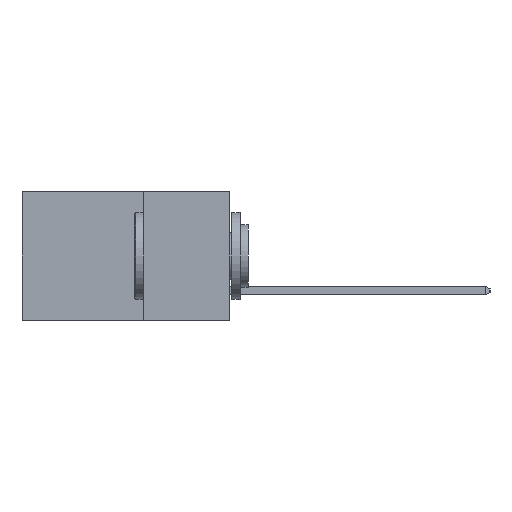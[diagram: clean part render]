
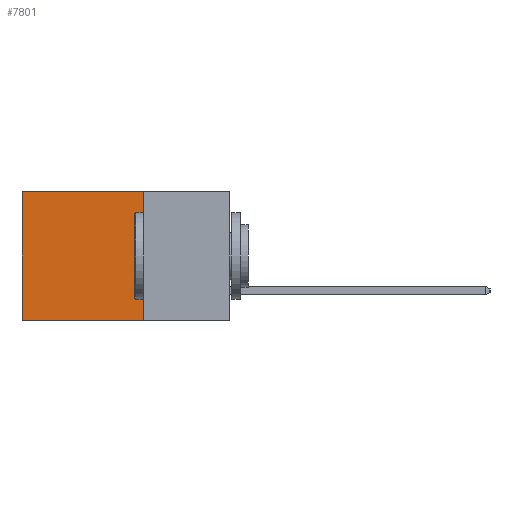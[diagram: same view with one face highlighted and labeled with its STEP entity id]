
A CAD part, left-side view. The second image highlights one B-rep face of the part: STEP entity #7801.
In plain terms, the highlighted planar face has unit normal (-1, 0, 0).
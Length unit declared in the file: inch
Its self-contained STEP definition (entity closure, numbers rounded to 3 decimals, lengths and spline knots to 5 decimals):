
#1 = LINE ( 'NONE', #16261, #3781 ) ;
#700 = ORIENTED_EDGE ( 'NONE', *, *, #13414, .F. ) ;
#1871 = ORIENTED_EDGE ( 'NONE', *, *, #15941, .T. ) ;
#2178 = CARTESIAN_POINT ( 'NONE',  ( 0.298, 0.25, 0. ) ) ;
#2342 = DIRECTION ( 'NONE',  ( 0., 0., -1. ) ) ;
#2393 = DIRECTION ( 'NONE',  ( 1., 0., 0. ) ) ;
#2459 = VECTOR ( 'NONE', #3857, 39.37008 ) ;
#2562 = CARTESIAN_POINT ( 'NONE',  ( 0.298, 0.25, 0. ) ) ;
#2691 = LINE ( 'NONE', #8338, #18317 ) ;
#3017 = PLANE ( 'NONE',  #8776 ) ;
#3781 = VECTOR ( 'NONE', #5329, 39.37008 ) ;
#3857 = DIRECTION ( 'NONE',  ( 0., 0., -1. ) ) ;
#3947 = CARTESIAN_POINT ( 'NONE',  ( 0.298, 0.6, 0. ) ) ;
#4878 = EDGE_LOOP ( 'NONE', ( #19168, #700, #9934, #1871 ) ) ;
#5329 = DIRECTION ( 'NONE',  ( 0., 1., 0. ) ) ;
#6420 = EDGE_CURVE ( 'NONE', #7809, #18587, #6676, .T. ) ;
#6676 = LINE ( 'NONE', #10028, #14474 ) ;
#7688 = EDGE_CURVE ( 'NONE', #8236, #14169, #10789, .T. ) ;
#7801 = ADVANCED_FACE ( 'NONE', ( #12972 ), #3017, .F. ) ;
#7809 = VERTEX_POINT ( 'NONE', #2178 ) ;
#8236 = VERTEX_POINT ( 'NONE', #13183 ) ;
#8338 = CARTESIAN_POINT ( 'NONE',  ( 0.298, 0.25, 0. ) ) ;
#8776 = AXIS2_PLACEMENT_3D ( 'NONE', #2562, #2393, #2342 ) ;
#9732 = DIRECTION ( 'NONE',  ( 0., 0., -1. ) ) ;
#9934 = ORIENTED_EDGE ( 'NONE', *, *, #6420, .F. ) ;
#10028 = CARTESIAN_POINT ( 'NONE',  ( 0.298, 0.25, 0. ) ) ;
#10789 = LINE ( 'NONE', #3947, #2459 ) ;
#12564 = CARTESIAN_POINT ( 'NONE',  ( 0.298, 0.25, -0.37 ) ) ;
#12972 = FACE_OUTER_BOUND ( 'NONE', #4878, .T. ) ;
#12977 = DIRECTION ( 'NONE',  ( 0., 1., 0. ) ) ;
#13183 = CARTESIAN_POINT ( 'NONE',  ( 0.298, 0.6, 0. ) ) ;
#13414 = EDGE_CURVE ( 'NONE', #18587, #14169, #1, .T. ) ;
#14169 = VERTEX_POINT ( 'NONE', #16463 ) ;
#14474 = VECTOR ( 'NONE', #9732, 39.37008 ) ;
#15941 = EDGE_CURVE ( 'NONE', #7809, #8236, #2691, .T. ) ;
#16261 = CARTESIAN_POINT ( 'NONE',  ( 0.298, 0.25, -0.37 ) ) ;
#16463 = CARTESIAN_POINT ( 'NONE',  ( 0.298, 0.6, -0.37 ) ) ;
#18317 = VECTOR ( 'NONE', #12977, 39.37008 ) ;
#18587 = VERTEX_POINT ( 'NONE', #12564 ) ;
#19168 = ORIENTED_EDGE ( 'NONE', *, *, #7688, .T. ) ;
